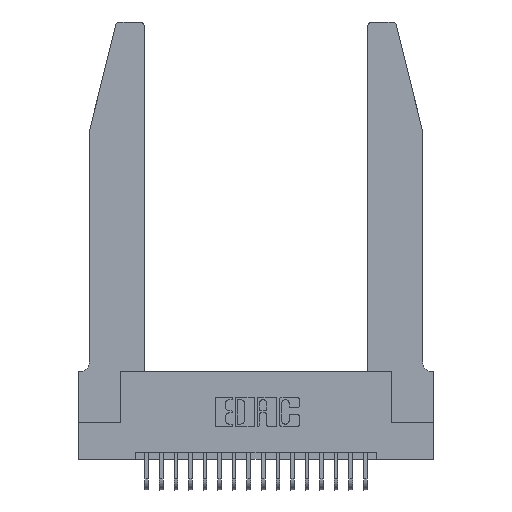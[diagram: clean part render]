
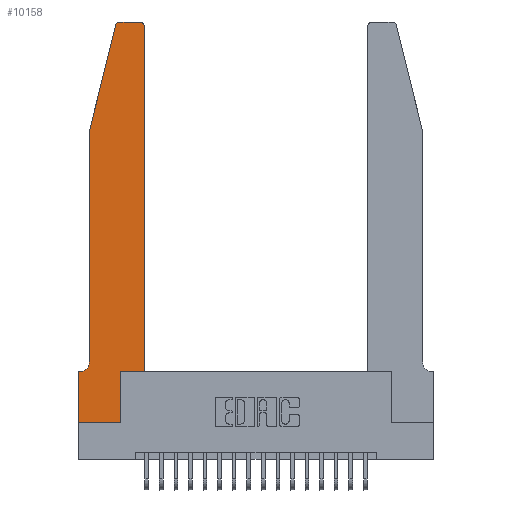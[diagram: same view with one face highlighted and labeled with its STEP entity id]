
A CAD part, top view. The second image highlights one B-rep face of the part: STEP entity #10158.
In plain terms, the highlighted planar face has unit normal (0, 0, 1).
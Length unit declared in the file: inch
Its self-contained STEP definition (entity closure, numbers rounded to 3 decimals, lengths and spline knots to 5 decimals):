
#53 = DIRECTION ( 'NONE',  ( 1., 0., 0. ) ) ;
#179 = CIRCLE ( 'NONE', #1677, 0.07 ) ;
#314 = CARTESIAN_POINT ( 'NONE',  ( 0.2865, 0., 0.37 ) ) ;
#348 = CARTESIAN_POINT ( 'NONE',  ( 0., 0.35, 0.37 ) ) ;
#586 = DIRECTION ( 'NONE',  ( -1., 0., 0. ) ) ;
#629 = VERTEX_POINT ( 'NONE', #19872 ) ;
#691 = CARTESIAN_POINT ( 'NONE',  ( 0.0055, 0.35, 0.37 ) ) ;
#815 = LINE ( 'NONE', #12873, #14207 ) ;
#839 = CARTESIAN_POINT ( 'NONE',  ( 0., 0., 0.37 ) ) ;
#1113 = LINE ( 'NONE', #6025, #10495 ) ;
#1481 = CARTESIAN_POINT ( 'NONE',  ( 0.4505, 0.35, 0.37 ) ) ;
#1677 = AXIS2_PLACEMENT_3D ( 'NONE', #20675, #10521, #22429 ) ;
#1811 = CARTESIAN_POINT ( 'NONE',  ( 0.25487, 2.72718, 0.37 ) ) ;
#2381 = DIRECTION ( 'NONE',  ( 0., -1., 0. ) ) ;
#2604 = LINE ( 'NONE', #21238, #15848 ) ;
#2651 = CARTESIAN_POINT ( 'NONE',  ( 0.4505, 0.35, 0.37 ) ) ;
#3314 = DIRECTION ( 'NONE',  ( 1., 0., 0. ) ) ;
#3651 = EDGE_CURVE ( 'NONE', #5859, #15223, #4112, .T. ) ;
#3680 = DIRECTION ( 'NONE',  ( 0., 1., 0. ) ) ;
#3789 = VERTEX_POINT ( 'NONE', #691 ) ;
#4112 = CIRCLE ( 'NONE', #4610, 0.03 ) ;
#4417 = LINE ( 'NONE', #839, #17523 ) ;
#4610 = AXIS2_PLACEMENT_3D ( 'NONE', #19361, #9240, #21106 ) ;
#4658 = ORIENTED_EDGE ( 'NONE', *, *, #5363, .T. ) ;
#4690 = CARTESIAN_POINT ( 'NONE',  ( 0.4505, 0.35, 0.37 ) ) ;
#5180 = EDGE_LOOP ( 'NONE', ( #16762, #5392, #12590, #11595, #22335, #7340, #17397, #17047, #14865, #21804, #4658, #10143 ) ) ;
#5363 = EDGE_CURVE ( 'NONE', #20124, #7695, #12736, .T. ) ;
#5392 = ORIENTED_EDGE ( 'NONE', *, *, #3651, .T. ) ;
#5859 = VERTEX_POINT ( 'NONE', #19378 ) ;
#5917 = EDGE_CURVE ( 'NONE', #15223, #9204, #16632, .T. ) ;
#6025 = CARTESIAN_POINT ( 'NONE',  ( 0.0755, 2., 0.37 ) ) ;
#6236 = CARTESIAN_POINT ( 'NONE',  ( 0.0755, 0.42, 0.37 ) ) ;
#7258 = CARTESIAN_POINT ( 'NONE',  ( 0.2865, 0.35, 0.37 ) ) ;
#7340 = ORIENTED_EDGE ( 'NONE', *, *, #13521, .T. ) ;
#7611 = VECTOR ( 'NONE', #21197, 39.37008 ) ;
#7687 = CARTESIAN_POINT ( 'NONE',  ( 0., 0., 0.37 ) ) ;
#7695 = VERTEX_POINT ( 'NONE', #22277 ) ;
#8111 = DIRECTION ( 'NONE',  ( 0., 0., 1. ) ) ;
#8154 = EDGE_CURVE ( 'NONE', #9204, #18880, #1113, .T. ) ;
#8726 = VECTOR ( 'NONE', #14756, 39.37008 ) ;
#8813 = AXIS2_PLACEMENT_3D ( 'NONE', #20810, #10672, #53 ) ;
#8956 = PLANE ( 'NONE',  #8813 ) ;
#9204 = VERTEX_POINT ( 'NONE', #12898 ) ;
#9240 = DIRECTION ( 'NONE',  ( 0., 0., 1. ) ) ;
#9415 = DIRECTION ( 'NONE',  ( -1., 0., 0. ) ) ;
#9768 = VERTEX_POINT ( 'NONE', #19619 ) ;
#10095 = EDGE_CURVE ( 'NONE', #18880, #3789, #179, .T. ) ;
#10143 = ORIENTED_EDGE ( 'NONE', *, *, #16385, .T. ) ;
#10158 = ADVANCED_FACE ( 'NONE', ( #22155 ), #8956, .T. ) ;
#10495 = VECTOR ( 'NONE', #16212, 39.37008 ) ;
#10521 = DIRECTION ( 'NONE',  ( 0., 0., -1. ) ) ;
#10672 = DIRECTION ( 'NONE',  ( 0., 0., 1. ) ) ;
#11332 = AXIS2_PLACEMENT_3D ( 'NONE', #18233, #8111, #19961 ) ;
#11595 = ORIENTED_EDGE ( 'NONE', *, *, #8154, .T. ) ;
#12590 = ORIENTED_EDGE ( 'NONE', *, *, #5917, .T. ) ;
#12659 = LINE ( 'NONE', #1481, #21101 ) ;
#12736 = LINE ( 'NONE', #2651, #8726 ) ;
#12761 = LINE ( 'NONE', #7687, #20677 ) ;
#12783 = CARTESIAN_POINT ( 'NONE',  ( 0.0755, 2., 0.37 ) ) ;
#12873 = CARTESIAN_POINT ( 'NONE',  ( 0.2605, 2.75, 0.37 ) ) ;
#12898 = CARTESIAN_POINT ( 'NONE',  ( 0.0755, 2., 0.37 ) ) ;
#13469 = VECTOR ( 'NONE', #3680, 39.37008 ) ;
#13521 = EDGE_CURVE ( 'NONE', #3789, #17899, #2604, .T. ) ;
#14207 = VECTOR ( 'NONE', #9415, 39.37008 ) ;
#14756 = DIRECTION ( 'NONE',  ( 0., 1., 0. ) ) ;
#14865 = ORIENTED_EDGE ( 'NONE', *, *, #15905, .T. ) ;
#15223 = VERTEX_POINT ( 'NONE', #1811 ) ;
#15848 = VECTOR ( 'NONE', #586, 39.37008 ) ;
#15905 = EDGE_CURVE ( 'NONE', #19838, #9768, #17360, .T. ) ;
#16059 = EDGE_CURVE ( 'NONE', #16580, #5859, #815, .T. ) ;
#16212 = DIRECTION ( 'NONE',  ( 0., -1., 0. ) ) ;
#16385 = EDGE_CURVE ( 'NONE', #7695, #16580, #21365, .T. ) ;
#16580 = VERTEX_POINT ( 'NONE', #17272 ) ;
#16632 = LINE ( 'NONE', #12783, #7611 ) ;
#16762 = ORIENTED_EDGE ( 'NONE', *, *, #16059, .T. ) ;
#17047 = ORIENTED_EDGE ( 'NONE', *, *, #18022, .T. ) ;
#17272 = CARTESIAN_POINT ( 'NONE',  ( 0.4205, 2.75, 0.37 ) ) ;
#17360 = LINE ( 'NONE', #7258, #13469 ) ;
#17397 = ORIENTED_EDGE ( 'NONE', *, *, #20499, .T. ) ;
#17523 = VECTOR ( 'NONE', #19880, 39.37008 ) ;
#17899 = VERTEX_POINT ( 'NONE', #348 ) ;
#18022 = EDGE_CURVE ( 'NONE', #629, #19838, #4417, .T. ) ;
#18233 = CARTESIAN_POINT ( 'NONE',  ( 0.4205, 2.72, 0.37 ) ) ;
#18880 = VERTEX_POINT ( 'NONE', #6236 ) ;
#19361 = CARTESIAN_POINT ( 'NONE',  ( 0.284, 2.72, 0.37 ) ) ;
#19378 = CARTESIAN_POINT ( 'NONE',  ( 0.284, 2.75, 0.37 ) ) ;
#19619 = CARTESIAN_POINT ( 'NONE',  ( 0.2865, 0.35, 0.37 ) ) ;
#19838 = VERTEX_POINT ( 'NONE', #314 ) ;
#19872 = CARTESIAN_POINT ( 'NONE',  ( 0., 0., 0.37 ) ) ;
#19880 = DIRECTION ( 'NONE',  ( 1., 0., 0. ) ) ;
#19961 = DIRECTION ( 'NONE',  ( 1., 0., 0. ) ) ;
#20124 = VERTEX_POINT ( 'NONE', #4690 ) ;
#20499 = EDGE_CURVE ( 'NONE', #17899, #629, #12761, .T. ) ;
#20675 = CARTESIAN_POINT ( 'NONE',  ( 0.0055, 0.42, 0.37 ) ) ;
#20677 = VECTOR ( 'NONE', #2381, 39.37008 ) ;
#20810 = CARTESIAN_POINT ( 'NONE',  ( 0., 0.35, 0.37 ) ) ;
#21101 = VECTOR ( 'NONE', #3314, 39.37008 ) ;
#21106 = DIRECTION ( 'NONE',  ( 1., 0., 0. ) ) ;
#21197 = DIRECTION ( 'NONE',  ( -0.239, -0.971, 0. ) ) ;
#21238 = CARTESIAN_POINT ( 'NONE',  ( 0.0755, 0.35, 0.37 ) ) ;
#21365 = CIRCLE ( 'NONE', #11332, 0.03 ) ;
#21804 = ORIENTED_EDGE ( 'NONE', *, *, #22198, .T. ) ;
#22155 = FACE_OUTER_BOUND ( 'NONE', #5180, .T. ) ;
#22198 = EDGE_CURVE ( 'NONE', #9768, #20124, #12659, .T. ) ;
#22277 = CARTESIAN_POINT ( 'NONE',  ( 0.4505, 2.72, 0.37 ) ) ;
#22335 = ORIENTED_EDGE ( 'NONE', *, *, #10095, .T. ) ;
#22429 = DIRECTION ( 'NONE',  ( -1., 0., 0. ) ) ;
